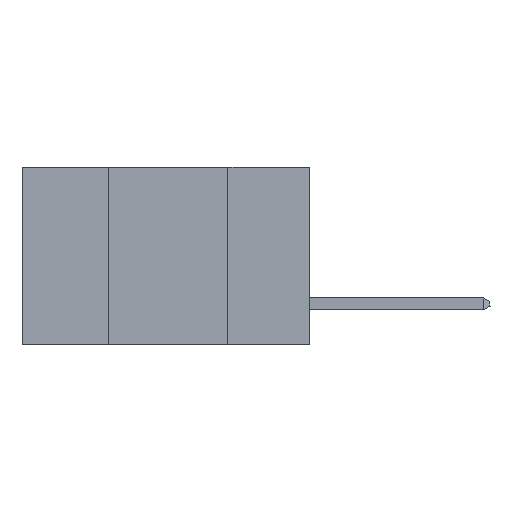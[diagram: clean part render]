
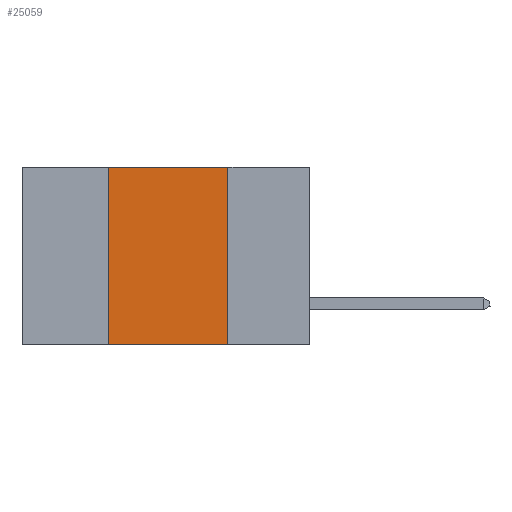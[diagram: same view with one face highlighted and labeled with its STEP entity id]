
A CAD part, left-side view. The second image highlights one B-rep face of the part: STEP entity #25059.
In plain terms, the highlighted planar face has unit normal (-1, 0, 0).
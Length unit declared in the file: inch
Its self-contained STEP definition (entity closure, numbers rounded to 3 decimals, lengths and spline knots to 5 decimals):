
#1551 = VERTEX_POINT ( 'NONE', #26417 ) ;
#1917 = EDGE_CURVE ( 'NONE', #42763, #15108, #28162, .T. ) ;
#3826 = VECTOR ( 'NONE', #40771, 39.37008 ) ;
#5518 = VECTOR ( 'NONE', #31654, 39.37008 ) ;
#6173 = VECTOR ( 'NONE', #18780, 39.37008 ) ;
#6418 = EDGE_CURVE ( 'NONE', #41815, #42763, #26040, .T. ) ;
#7769 = AXIS2_PLACEMENT_3D ( 'NONE', #29627, #19789, #30368 ) ;
#8387 = CARTESIAN_POINT ( 'NONE',  ( 0., 0.6, -0.37 ) ) ;
#8551 = CARTESIAN_POINT ( 'NONE',  ( 0., 0.42, 0. ) ) ;
#12033 = DIRECTION ( 'NONE',  ( 0., -1., 0. ) ) ;
#13740 = LINE ( 'NONE', #41910, #6173 ) ;
#15108 = VERTEX_POINT ( 'NONE', #25793 ) ;
#16414 = EDGE_LOOP ( 'NONE', ( #39397, #29791, #31039, #40674 ) ) ;
#18780 = DIRECTION ( 'NONE',  ( 0., 0., -1. ) ) ;
#19789 = DIRECTION ( 'NONE',  ( 1., 0., 0. ) ) ;
#20708 = VECTOR ( 'NONE', #12033, 39.37008 ) ;
#22371 = FACE_OUTER_BOUND ( 'NONE', #16414, .T. ) ;
#24744 = CARTESIAN_POINT ( 'NONE',  ( 0., 0.42, 0. ) ) ;
#25059 = ADVANCED_FACE ( 'NONE', ( #22371 ), #32181, .F. ) ;
#25793 = CARTESIAN_POINT ( 'NONE',  ( 0., 0.17, 0. ) ) ;
#26040 = LINE ( 'NONE', #24744, #5518 ) ;
#26417 = CARTESIAN_POINT ( 'NONE',  ( 0., 0.17, -0.37 ) ) ;
#28162 = LINE ( 'NONE', #33841, #3826 ) ;
#29627 = CARTESIAN_POINT ( 'NONE',  ( 0., 0.6, 0. ) ) ;
#29791 = ORIENTED_EDGE ( 'NONE', *, *, #1917, .F. ) ;
#30368 = DIRECTION ( 'NONE',  ( 0., 0., -1. ) ) ;
#30494 = CARTESIAN_POINT ( 'NONE',  ( 0., 0.42, -0.37 ) ) ;
#31039 = ORIENTED_EDGE ( 'NONE', *, *, #6418, .F. ) ;
#31654 = DIRECTION ( 'NONE',  ( 0., 0., 1. ) ) ;
#32181 = PLANE ( 'NONE',  #7769 ) ;
#33841 = CARTESIAN_POINT ( 'NONE',  ( 0., 0.6, 0. ) ) ;
#36874 = EDGE_CURVE ( 'NONE', #15108, #1551, #13740, .T. ) ;
#36919 = EDGE_CURVE ( 'NONE', #41815, #1551, #39082, .T. ) ;
#39082 = LINE ( 'NONE', #8387, #20708 ) ;
#39397 = ORIENTED_EDGE ( 'NONE', *, *, #36874, .F. ) ;
#40674 = ORIENTED_EDGE ( 'NONE', *, *, #36919, .T. ) ;
#40771 = DIRECTION ( 'NONE',  ( 0., -1., 0. ) ) ;
#41815 = VERTEX_POINT ( 'NONE', #30494 ) ;
#41910 = CARTESIAN_POINT ( 'NONE',  ( 0., 0.17, 0. ) ) ;
#42763 = VERTEX_POINT ( 'NONE', #8551 ) ;
